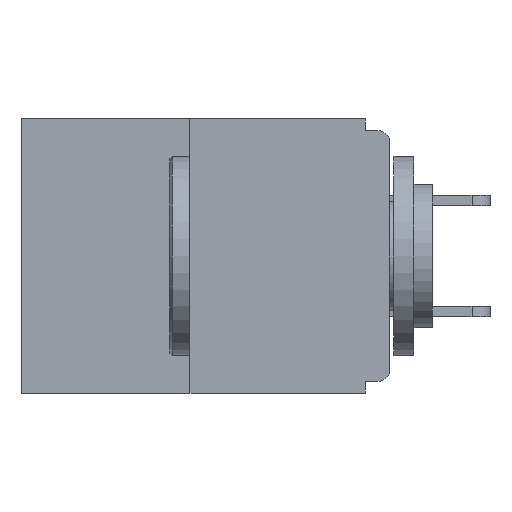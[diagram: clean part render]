
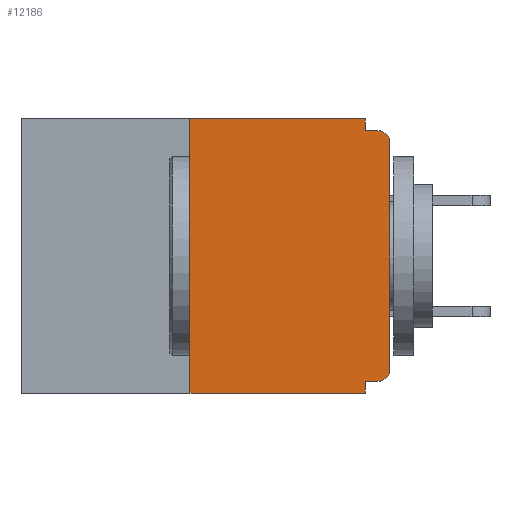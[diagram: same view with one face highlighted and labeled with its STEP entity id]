
A CAD part, left-side view. The second image highlights one B-rep face of the part: STEP entity #12186.
In plain terms, the highlighted planar face has unit normal (-1, 0, 0).
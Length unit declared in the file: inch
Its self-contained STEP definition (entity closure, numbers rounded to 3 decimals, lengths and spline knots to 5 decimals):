
#1 = CIRCLE ( 'NONE', #12322, 0.015 ) ;
#388 = FACE_OUTER_BOUND ( 'NONE', #16806, .T. ) ;
#704 = ORIENTED_EDGE ( 'NONE', *, *, #3341, .F. ) ;
#785 = DIRECTION ( 'NONE',  ( 1., 0., 0. ) ) ;
#966 = CARTESIAN_POINT ( 'NONE',  ( 0., 0.46, 0. ) ) ;
#1093 = EDGE_CURVE ( 'NONE', #16584, #20401, #12019, .T. ) ;
#1236 = EDGE_CURVE ( 'NONE', #9016, #20242, #9806, .T. ) ;
#1250 = DIRECTION ( 'NONE',  ( 0., -1., 0. ) ) ;
#1784 = EDGE_CURVE ( 'NONE', #8429, #2180, #4833, .T. ) ;
#1790 = CARTESIAN_POINT ( 'NONE',  ( 0., 0.25, -0.343 ) ) ;
#2180 = VERTEX_POINT ( 'NONE', #10909 ) ;
#2567 = DIRECTION ( 'NONE',  ( 0., 1., 0. ) ) ;
#3269 = VECTOR ( 'NONE', #1250, 39.37008 ) ;
#3321 = EDGE_CURVE ( 'NONE', #15745, #8429, #7208, .T. ) ;
#3341 = EDGE_CURVE ( 'NONE', #6682, #8228, #10939, .T. ) ;
#3343 = CARTESIAN_POINT ( 'NONE',  ( 0., 0.015, -0.03 ) ) ;
#3640 = CARTESIAN_POINT ( 'NONE',  ( 0., 0.25, 0. ) ) ;
#3844 = VECTOR ( 'NONE', #20359, 39.37008 ) ;
#4135 = ORIENTED_EDGE ( 'NONE', *, *, #11952, .F. ) ;
#4400 = CARTESIAN_POINT ( 'NONE',  ( 0., 0.031, -0.343 ) ) ;
#4766 = VERTEX_POINT ( 'NONE', #19334 ) ;
#4833 = LINE ( 'NONE', #15734, #12781 ) ;
#5061 = DIRECTION ( 'NONE',  ( -1., 0., 0. ) ) ;
#5124 = DIRECTION ( 'NONE',  ( -1., 0., 0. ) ) ;
#5786 = CARTESIAN_POINT ( 'NONE',  ( 0., 0.031, -0.328 ) ) ;
#6682 = VERTEX_POINT ( 'NONE', #12209 ) ;
#7203 = DIRECTION ( 'NONE',  ( 0., 0., 1. ) ) ;
#7208 = LINE ( 'NONE', #966, #3269 ) ;
#7293 = AXIS2_PLACEMENT_3D ( 'NONE', #8691, #785, #13461 ) ;
#7537 = ORIENTED_EDGE ( 'NONE', *, *, #1236, .T. ) ;
#7721 = CARTESIAN_POINT ( 'NONE',  ( 0., 0.031, 0. ) ) ;
#7947 = ORIENTED_EDGE ( 'NONE', *, *, #7951, .T. ) ;
#7951 = EDGE_CURVE ( 'NONE', #20401, #4766, #17858, .T. ) ;
#8228 = VERTEX_POINT ( 'NONE', #5786 ) ;
#8429 = VERTEX_POINT ( 'NONE', #7721 ) ;
#8691 = CARTESIAN_POINT ( 'NONE',  ( 0., 0.46, 0. ) ) ;
#8808 = VECTOR ( 'NONE', #7203, 39.37008 ) ;
#8908 = DIRECTION ( 'NONE',  ( 0., 0., -1. ) ) ;
#9016 = VERTEX_POINT ( 'NONE', #1790 ) ;
#9415 = EDGE_CURVE ( 'NONE', #6682, #16584, #1, .T. ) ;
#9420 = DIRECTION ( 'NONE',  ( 0., 0., -1. ) ) ;
#9725 = ORIENTED_EDGE ( 'NONE', *, *, #20407, .F. ) ;
#9806 = LINE ( 'NONE', #12341, #3844 ) ;
#10062 = LINE ( 'NONE', #4400, #15018 ) ;
#10246 = CARTESIAN_POINT ( 'NONE',  ( 0., 0., -0.313 ) ) ;
#10841 = ORIENTED_EDGE ( 'NONE', *, *, #14790, .F. ) ;
#10909 = CARTESIAN_POINT ( 'NONE',  ( 0., 0.031, -0.015 ) ) ;
#10939 = LINE ( 'NONE', #12041, #15153 ) ;
#11952 = EDGE_CURVE ( 'NONE', #9016, #15745, #16503, .T. ) ;
#12019 = LINE ( 'NONE', #20010, #8808 ) ;
#12041 = CARTESIAN_POINT ( 'NONE',  ( 0., 0., -0.328 ) ) ;
#12186 = ADVANCED_FACE ( 'NONE', ( #388 ), #18175, .F. ) ;
#12209 = CARTESIAN_POINT ( 'NONE',  ( 0., 0.015, -0.328 ) ) ;
#12322 = AXIS2_PLACEMENT_3D ( 'NONE', #17749, #5124, #16214 ) ;
#12341 = CARTESIAN_POINT ( 'NONE',  ( 0., 0.46, -0.343 ) ) ;
#12781 = VECTOR ( 'NONE', #9420, 39.37008 ) ;
#13136 = LINE ( 'NONE', #16232, #14880 ) ;
#13461 = DIRECTION ( 'NONE',  ( 0., 0., -1. ) ) ;
#14499 = DIRECTION ( 'NONE',  ( 0., 0., -1. ) ) ;
#14790 = EDGE_CURVE ( 'NONE', #2180, #4766, #13136, .T. ) ;
#14880 = VECTOR ( 'NONE', #17697, 39.37008 ) ;
#15018 = VECTOR ( 'NONE', #8908, 39.37008 ) ;
#15153 = VECTOR ( 'NONE', #2567, 39.37008 ) ;
#15734 = CARTESIAN_POINT ( 'NONE',  ( 0., 0.031, 0. ) ) ;
#15745 = VERTEX_POINT ( 'NONE', #18632 ) ;
#15827 = CARTESIAN_POINT ( 'NONE',  ( 0., 0.031, -0.343 ) ) ;
#15851 = ORIENTED_EDGE ( 'NONE', *, *, #1093, .T. ) ;
#16214 = DIRECTION ( 'NONE',  ( 0., 0., -1. ) ) ;
#16232 = CARTESIAN_POINT ( 'NONE',  ( 0., 0., -0.015 ) ) ;
#16503 = LINE ( 'NONE', #3640, #19458 ) ;
#16578 = ORIENTED_EDGE ( 'NONE', *, *, #9415, .T. ) ;
#16584 = VERTEX_POINT ( 'NONE', #10246 ) ;
#16806 = EDGE_LOOP ( 'NONE', ( #18988, #4135, #7537, #9725, #704, #16578, #15851, #7947, #10841, #19660 ) ) ;
#17697 = DIRECTION ( 'NONE',  ( 0., -1., 0. ) ) ;
#17749 = CARTESIAN_POINT ( 'NONE',  ( 0., 0.015, -0.313 ) ) ;
#17858 = CIRCLE ( 'NONE', #18157, 0.015 ) ;
#18157 = AXIS2_PLACEMENT_3D ( 'NONE', #3343, #5061, #14499 ) ;
#18175 = PLANE ( 'NONE',  #7293 ) ;
#18632 = CARTESIAN_POINT ( 'NONE',  ( 0., 0.25, 0. ) ) ;
#18988 = ORIENTED_EDGE ( 'NONE', *, *, #3321, .F. ) ;
#19222 = DIRECTION ( 'NONE',  ( 0., 0., 1. ) ) ;
#19334 = CARTESIAN_POINT ( 'NONE',  ( 0., 0.015, -0.015 ) ) ;
#19458 = VECTOR ( 'NONE', #19222, 39.37008 ) ;
#19660 = ORIENTED_EDGE ( 'NONE', *, *, #1784, .F. ) ;
#20010 = CARTESIAN_POINT ( 'NONE',  ( 0., 0., 0. ) ) ;
#20180 = CARTESIAN_POINT ( 'NONE',  ( 0., 0., -0.03 ) ) ;
#20242 = VERTEX_POINT ( 'NONE', #15827 ) ;
#20359 = DIRECTION ( 'NONE',  ( 0., -1., 0. ) ) ;
#20401 = VERTEX_POINT ( 'NONE', #20180 ) ;
#20407 = EDGE_CURVE ( 'NONE', #8228, #20242, #10062, .T. ) ;
